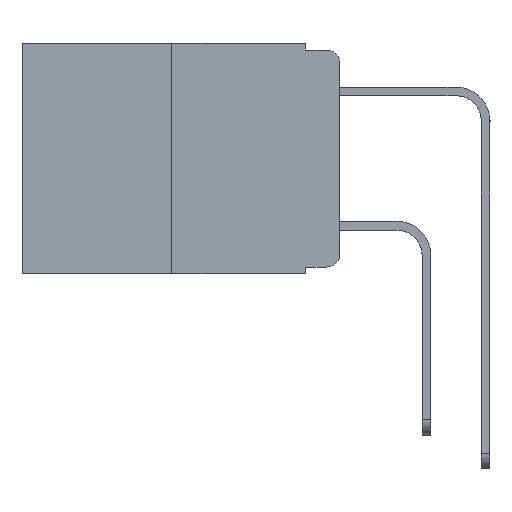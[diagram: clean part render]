
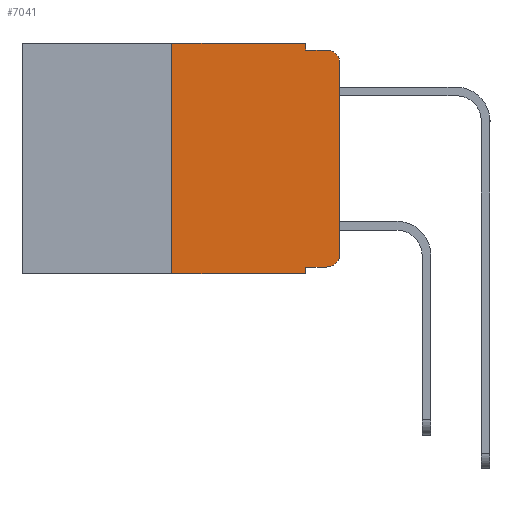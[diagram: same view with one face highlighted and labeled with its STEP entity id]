
A CAD part, left-side view. The second image highlights one B-rep face of the part: STEP entity #7041.
In plain terms, the highlighted planar face has unit normal (-1, 0, 0).
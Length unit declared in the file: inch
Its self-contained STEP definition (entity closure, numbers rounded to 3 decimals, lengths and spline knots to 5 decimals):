
#73 = LINE ( 'NONE', #486, #3782 ) ;
#238 = PLANE ( 'NONE',  #4046 ) ;
#381 = CARTESIAN_POINT ( 'NONE',  ( 0., 0.051, -0.343 ) ) ;
#423 = EDGE_CURVE ( 'NONE', #1093, #7096, #73, .T. ) ;
#486 = CARTESIAN_POINT ( 'NONE',  ( 0., 0.051, 0. ) ) ;
#611 = DIRECTION ( 'NONE',  ( 0., 0., 1. ) ) ;
#999 = ORIENTED_EDGE ( 'NONE', *, *, #423, .F. ) ;
#1093 = VERTEX_POINT ( 'NONE', #9722 ) ;
#1511 = EDGE_CURVE ( 'NONE', #14871, #3993, #6341, .T. ) ;
#1610 = DIRECTION ( 'NONE',  ( 0., 0., -1. ) ) ;
#1860 = DIRECTION ( 'NONE',  ( 1., 0., 0. ) ) ;
#1919 = CARTESIAN_POINT ( 'NONE',  ( 0., 0.473, 0. ) ) ;
#2196 = CARTESIAN_POINT ( 'NONE',  ( 0., 0.051, 0. ) ) ;
#2559 = EDGE_CURVE ( 'NONE', #8465, #16522, #18772, .T. ) ;
#2810 = CIRCLE ( 'NONE', #2821, 0.02 ) ;
#2821 = AXIS2_PLACEMENT_3D ( 'NONE', #7434, #17380, #8900 ) ;
#2868 = DIRECTION ( 'NONE',  ( -1., 0., 0. ) ) ;
#3192 = DIRECTION ( 'NONE',  ( 0., 0., -1. ) ) ;
#3208 = ORIENTED_EDGE ( 'NONE', *, *, #3601, .F. ) ;
#3275 = VERTEX_POINT ( 'NONE', #13522 ) ;
#3601 = EDGE_CURVE ( 'NONE', #16522, #11048, #14603, .T. ) ;
#3782 = VECTOR ( 'NONE', #1610, 39.37008 ) ;
#3904 = CARTESIAN_POINT ( 'NONE',  ( 0., 0.051, -0.01 ) ) ;
#3993 = VERTEX_POINT ( 'NONE', #15052 ) ;
#4046 = AXIS2_PLACEMENT_3D ( 'NONE', #10786, #1860, #12193 ) ;
#4180 = ORIENTED_EDGE ( 'NONE', *, *, #1511, .F. ) ;
#5142 = ORIENTED_EDGE ( 'NONE', *, *, #18458, .T. ) ;
#5618 = ORIENTED_EDGE ( 'NONE', *, *, #17541, .T. ) ;
#5658 = EDGE_CURVE ( 'NONE', #3275, #11048, #2810, .T. ) ;
#5927 = CARTESIAN_POINT ( 'NONE',  ( 0., 0.051, -0.01 ) ) ;
#6315 = CARTESIAN_POINT ( 'NONE',  ( 0., 0.02, -0.333 ) ) ;
#6341 = LINE ( 'NONE', #15768, #13106 ) ;
#6607 = AXIS2_PLACEMENT_3D ( 'NONE', #11698, #2868, #13167 ) ;
#6610 = VECTOR ( 'NONE', #12252, 39.37008 ) ;
#6657 = EDGE_CURVE ( 'NONE', #15652, #3275, #17573, .T. ) ;
#6772 = ORIENTED_EDGE ( 'NONE', *, *, #6657, .T. ) ;
#6816 = VECTOR ( 'NONE', #14071, 39.37008 ) ;
#7041 = ADVANCED_FACE ( 'NONE', ( #7086 ), #238, .F. ) ;
#7065 = EDGE_CURVE ( 'NONE', #3993, #8465, #17555, .T. ) ;
#7086 = FACE_OUTER_BOUND ( 'NONE', #18667, .T. ) ;
#7096 = VERTEX_POINT ( 'NONE', #381 ) ;
#7308 = LINE ( 'NONE', #12587, #6816 ) ;
#7316 = CARTESIAN_POINT ( 'NONE',  ( 0., 0.473, -0.343 ) ) ;
#7434 = CARTESIAN_POINT ( 'NONE',  ( 0., 0.02, -0.03 ) ) ;
#7715 = VERTEX_POINT ( 'NONE', #6315 ) ;
#7734 = ORIENTED_EDGE ( 'NONE', *, *, #7065, .F. ) ;
#7997 = CARTESIAN_POINT ( 'NONE',  ( 0., 0.051, 0. ) ) ;
#8258 = CARTESIAN_POINT ( 'NONE',  ( 0., 0., 0. ) ) ;
#8390 = VECTOR ( 'NONE', #3192, 39.37008 ) ;
#8465 = VERTEX_POINT ( 'NONE', #7997 ) ;
#8900 = DIRECTION ( 'NONE',  ( 0., 0., -1. ) ) ;
#9619 = VECTOR ( 'NONE', #611, 39.37008 ) ;
#9722 = CARTESIAN_POINT ( 'NONE',  ( 0., 0.051, -0.333 ) ) ;
#10201 = EDGE_CURVE ( 'NONE', #14871, #7096, #14637, .T. ) ;
#10625 = ORIENTED_EDGE ( 'NONE', *, *, #5658, .T. ) ;
#10786 = CARTESIAN_POINT ( 'NONE',  ( 0., 0.473, 0. ) ) ;
#10935 = CARTESIAN_POINT ( 'NONE',  ( 0., 0.25, -0.343 ) ) ;
#11048 = VERTEX_POINT ( 'NONE', #17540 ) ;
#11054 = ORIENTED_EDGE ( 'NONE', *, *, #2559, .F. ) ;
#11190 = CARTESIAN_POINT ( 'NONE',  ( 0., 0., -0.313 ) ) ;
#11219 = VECTOR ( 'NONE', #15566, 39.37008 ) ;
#11323 = CIRCLE ( 'NONE', #6607, 0.02 ) ;
#11698 = CARTESIAN_POINT ( 'NONE',  ( 0., 0.02, -0.313 ) ) ;
#12193 = DIRECTION ( 'NONE',  ( 0., 0., -1. ) ) ;
#12252 = DIRECTION ( 'NONE',  ( 0., -1., 0. ) ) ;
#12366 = ORIENTED_EDGE ( 'NONE', *, *, #10201, .T. ) ;
#12587 = CARTESIAN_POINT ( 'NONE',  ( 0., 0.051, -0.333 ) ) ;
#13106 = VECTOR ( 'NONE', #15832, 39.37008 ) ;
#13167 = DIRECTION ( 'NONE',  ( 0., 0., -1. ) ) ;
#13522 = CARTESIAN_POINT ( 'NONE',  ( 0., 0., -0.03 ) ) ;
#14071 = DIRECTION ( 'NONE',  ( 0., -1., 0. ) ) ;
#14445 = DIRECTION ( 'NONE',  ( 0., -1., 0. ) ) ;
#14603 = LINE ( 'NONE', #3904, #11219 ) ;
#14637 = LINE ( 'NONE', #7316, #18335 ) ;
#14871 = VERTEX_POINT ( 'NONE', #10935 ) ;
#15052 = CARTESIAN_POINT ( 'NONE',  ( 0., 0.25, 0. ) ) ;
#15566 = DIRECTION ( 'NONE',  ( 0., -1., 0. ) ) ;
#15652 = VERTEX_POINT ( 'NONE', #11190 ) ;
#15768 = CARTESIAN_POINT ( 'NONE',  ( 0., 0.25, 0. ) ) ;
#15832 = DIRECTION ( 'NONE',  ( 0., 0., 1. ) ) ;
#16522 = VERTEX_POINT ( 'NONE', #5927 ) ;
#17380 = DIRECTION ( 'NONE',  ( -1., 0., 0. ) ) ;
#17540 = CARTESIAN_POINT ( 'NONE',  ( 0., 0.02, -0.01 ) ) ;
#17541 = EDGE_CURVE ( 'NONE', #7715, #15652, #11323, .T. ) ;
#17555 = LINE ( 'NONE', #1919, #6610 ) ;
#17573 = LINE ( 'NONE', #8258, #9619 ) ;
#18335 = VECTOR ( 'NONE', #14445, 39.37008 ) ;
#18458 = EDGE_CURVE ( 'NONE', #1093, #7715, #7308, .T. ) ;
#18667 = EDGE_LOOP ( 'NONE', ( #6772, #10625, #3208, #11054, #7734, #4180, #12366, #999, #5142, #5618 ) ) ;
#18772 = LINE ( 'NONE', #2196, #8390 ) ;
